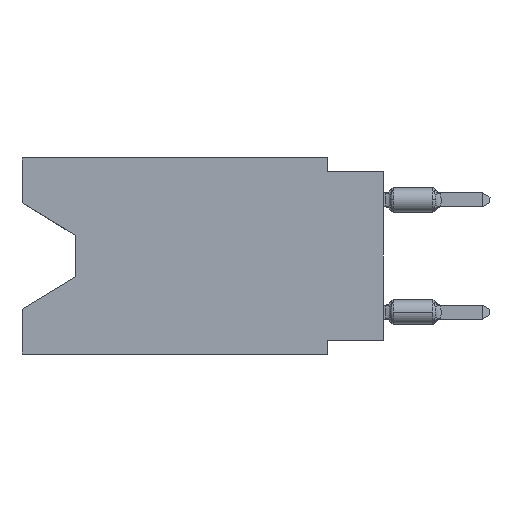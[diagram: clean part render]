
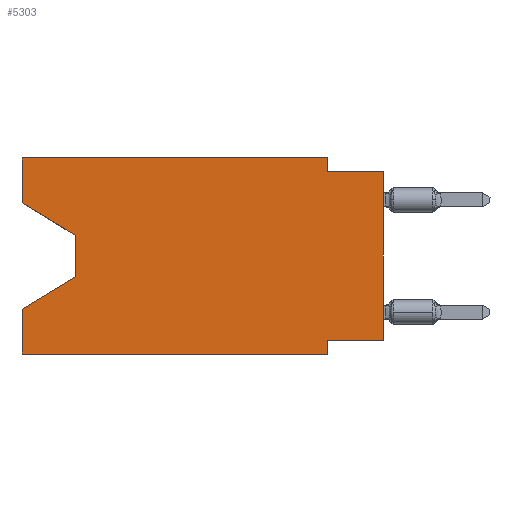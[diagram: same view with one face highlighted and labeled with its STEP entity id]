
A CAD part, left-side view. The second image highlights one B-rep face of the part: STEP entity #5303.
In plain terms, the highlighted planar face has unit normal (-1, 0, 0).
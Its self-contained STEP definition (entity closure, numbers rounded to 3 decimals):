
#34 = LINE ( 'NONE', #8749, #17924 ) ;
#64 = EDGE_CURVE ( 'NONE', #12275, #13794, #7933, .T. ) ;
#89 = VECTOR ( 'NONE', #784, 1000. ) ;
#158 = EDGE_CURVE ( 'NONE', #5256, #1109, #6937, .T. ) ;
#264 = ORIENTED_EDGE ( 'NONE', *, *, #6274, .F. ) ;
#480 = CARTESIAN_POINT ( 'NONE',  ( 0., 2.54, -8.89 ) ) ;
#640 = DIRECTION ( 'NONE',  ( 0., 0., -1. ) ) ;
#718 = CARTESIAN_POINT ( 'NONE',  ( 0., 2.54, -0.635 ) ) ;
#784 = DIRECTION ( 'NONE',  ( 0., 0., 1. ) ) ;
#824 = LINE ( 'NONE', #3709, #8961 ) ;
#933 = DIRECTION ( 'NONE',  ( 0., -1., 0. ) ) ;
#1070 = ORIENTED_EDGE ( 'NONE', *, *, #4562, .F. ) ;
#1109 = VERTEX_POINT ( 'NONE', #3903 ) ;
#1167 = DIRECTION ( 'NONE',  ( 0., -1., 0. ) ) ;
#1632 = AXIS2_PLACEMENT_3D ( 'NONE', #11495, #5327, #640 ) ;
#2377 = DIRECTION ( 'NONE',  ( 0., 0., -1. ) ) ;
#2695 = CARTESIAN_POINT ( 'NONE',  ( 0., 0., -0.635 ) ) ;
#2892 = LINE ( 'NONE', #19076, #12207 ) ;
#2978 = CARTESIAN_POINT ( 'NONE',  ( 0., 2.54, -8.255 ) ) ;
#3709 = CARTESIAN_POINT ( 'NONE',  ( 0., 16.383, 0. ) ) ;
#3861 = CARTESIAN_POINT ( 'NONE',  ( 0., 13.97, -3.505 ) ) ;
#3863 = CARTESIAN_POINT ( 'NONE',  ( 0., 0., 0. ) ) ;
#3903 = CARTESIAN_POINT ( 'NONE',  ( 0., 2.54, -8.89 ) ) ;
#4438 = EDGE_CURVE ( 'NONE', #8573, #5256, #6000, .T. ) ;
#4557 = VECTOR ( 'NONE', #1167, 1000. ) ;
#4562 = EDGE_CURVE ( 'NONE', #18750, #13744, #824, .T. ) ;
#4615 = VERTEX_POINT ( 'NONE', #718 ) ;
#4851 = CARTESIAN_POINT ( 'NONE',  ( 0., 13.97, -5.385 ) ) ;
#5234 = PLANE ( 'NONE',  #1632 ) ;
#5256 = VERTEX_POINT ( 'NONE', #2978 ) ;
#5257 = CARTESIAN_POINT ( 'NONE',  ( 0., 13.97, -5.385 ) ) ;
#5303 = ADVANCED_FACE ( 'NONE', ( #9806 ), #5234, .F. ) ;
#5327 = DIRECTION ( 'NONE',  ( 1., 0., 0. ) ) ;
#5358 = LINE ( 'NONE', #8345, #11338 ) ;
#5850 = VECTOR ( 'NONE', #18910, 1000. ) ;
#6000 = LINE ( 'NONE', #12372, #19156 ) ;
#6045 = CARTESIAN_POINT ( 'NONE',  ( 0., 13.97, -3.505 ) ) ;
#6274 = EDGE_CURVE ( 'NONE', #4615, #19054, #12311, .T. ) ;
#6423 = VECTOR ( 'NONE', #11707, 1000. ) ;
#6498 = DIRECTION ( 'NONE',  ( 0., 0., 1. ) ) ;
#6937 = LINE ( 'NONE', #480, #5850 ) ;
#7058 = CARTESIAN_POINT ( 'NONE',  ( 0., 16.383, -6.852 ) ) ;
#7338 = EDGE_CURVE ( 'NONE', #18586, #4615, #5358, .T. ) ;
#7933 = LINE ( 'NONE', #6045, #17004 ) ;
#8258 = ORIENTED_EDGE ( 'NONE', *, *, #13332, .F. ) ;
#8322 = VERTEX_POINT ( 'NONE', #18266 ) ;
#8345 = CARTESIAN_POINT ( 'NONE',  ( 0., 2.54, 0. ) ) ;
#8573 = VERTEX_POINT ( 'NONE', #19242 ) ;
#8749 = CARTESIAN_POINT ( 'NONE',  ( 0., 16.383, 0. ) ) ;
#8818 = EDGE_CURVE ( 'NONE', #8573, #19054, #14534, .T. ) ;
#8961 = VECTOR ( 'NONE', #6498, 1000. ) ;
#8978 = EDGE_CURVE ( 'NONE', #8322, #14650, #34, .T. ) ;
#9230 = DIRECTION ( 'NONE',  ( 0., 0., -1. ) ) ;
#9262 = VECTOR ( 'NONE', #12511, 1000. ) ;
#9541 = LINE ( 'NONE', #11142, #6423 ) ;
#9738 = CARTESIAN_POINT ( 'NONE',  ( 0., 16.383, 0. ) ) ;
#9806 = FACE_OUTER_BOUND ( 'NONE', #12747, .T. ) ;
#11142 = CARTESIAN_POINT ( 'NONE',  ( 0., 16.383, -2.038 ) ) ;
#11335 = DIRECTION ( 'NONE',  ( 0., 0.855, -0.519 ) ) ;
#11338 = VECTOR ( 'NONE', #2377, 1000. ) ;
#11495 = CARTESIAN_POINT ( 'NONE',  ( 0., 16.383, 0. ) ) ;
#11511 = ORIENTED_EDGE ( 'NONE', *, *, #64, .T. ) ;
#11707 = DIRECTION ( 'NONE',  ( 0., -0.855, -0.519 ) ) ;
#12207 = VECTOR ( 'NONE', #933, 1000. ) ;
#12275 = VERTEX_POINT ( 'NONE', #3861 ) ;
#12311 = LINE ( 'NONE', #15506, #9262 ) ;
#12372 = CARTESIAN_POINT ( 'NONE',  ( 0., 0., -8.255 ) ) ;
#12511 = DIRECTION ( 'NONE',  ( 0., -1., 0. ) ) ;
#12531 = ORIENTED_EDGE ( 'NONE', *, *, #4438, .F. ) ;
#12625 = ORIENTED_EDGE ( 'NONE', *, *, #8978, .F. ) ;
#12747 = EDGE_LOOP ( 'NONE', ( #15211, #11511, #19294, #12625, #13385, #13966, #12531, #13666, #264, #14537, #8258, #1070 ) ) ;
#13332 = EDGE_CURVE ( 'NONE', #13744, #18586, #15548, .T. ) ;
#13385 = ORIENTED_EDGE ( 'NONE', *, *, #14230, .T. ) ;
#13666 = ORIENTED_EDGE ( 'NONE', *, *, #8818, .T. ) ;
#13744 = VERTEX_POINT ( 'NONE', #9738 ) ;
#13794 = VERTEX_POINT ( 'NONE', #4851 ) ;
#13837 = VECTOR ( 'NONE', #11335, 1000. ) ;
#13966 = ORIENTED_EDGE ( 'NONE', *, *, #158, .F. ) ;
#14047 = CARTESIAN_POINT ( 'NONE',  ( 0., 16.383, 0. ) ) ;
#14230 = EDGE_CURVE ( 'NONE', #8322, #1109, #2892, .T. ) ;
#14276 = CARTESIAN_POINT ( 'NONE',  ( 0., 2.54, 0. ) ) ;
#14534 = LINE ( 'NONE', #3863, #89 ) ;
#14537 = ORIENTED_EDGE ( 'NONE', *, *, #7338, .F. ) ;
#14650 = VERTEX_POINT ( 'NONE', #7058 ) ;
#14823 = DIRECTION ( 'NONE',  ( 0., 0., 1. ) ) ;
#15023 = EDGE_CURVE ( 'NONE', #13794, #14650, #18914, .T. ) ;
#15211 = ORIENTED_EDGE ( 'NONE', *, *, #19308, .T. ) ;
#15250 = CARTESIAN_POINT ( 'NONE',  ( 0., 16.383, -2.038 ) ) ;
#15506 = CARTESIAN_POINT ( 'NONE',  ( 0., 0., -0.635 ) ) ;
#15548 = LINE ( 'NONE', #14047, #4557 ) ;
#17004 = VECTOR ( 'NONE', #9230, 1000. ) ;
#17924 = VECTOR ( 'NONE', #14823, 1000. ) ;
#18266 = CARTESIAN_POINT ( 'NONE',  ( 0., 16.383, -8.89 ) ) ;
#18565 = DIRECTION ( 'NONE',  ( 0., 1., 0. ) ) ;
#18586 = VERTEX_POINT ( 'NONE', #14276 ) ;
#18750 = VERTEX_POINT ( 'NONE', #15250 ) ;
#18910 = DIRECTION ( 'NONE',  ( 0., 0., -1. ) ) ;
#18914 = LINE ( 'NONE', #5257, #13837 ) ;
#19054 = VERTEX_POINT ( 'NONE', #2695 ) ;
#19076 = CARTESIAN_POINT ( 'NONE',  ( 0., 16.383, -8.89 ) ) ;
#19156 = VECTOR ( 'NONE', #18565, 1000. ) ;
#19242 = CARTESIAN_POINT ( 'NONE',  ( 0., 0., -8.255 ) ) ;
#19294 = ORIENTED_EDGE ( 'NONE', *, *, #15023, .T. ) ;
#19308 = EDGE_CURVE ( 'NONE', #18750, #12275, #9541, .T. ) ;
